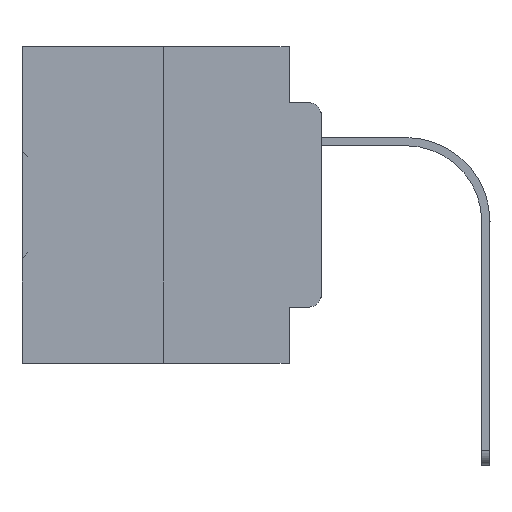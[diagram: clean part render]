
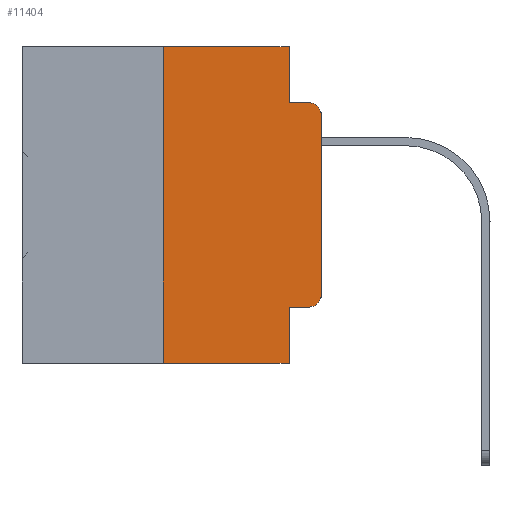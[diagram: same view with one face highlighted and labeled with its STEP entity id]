
A CAD part, left-side view. The second image highlights one B-rep face of the part: STEP entity #11404.
In plain terms, the highlighted planar face has unit normal (-1, 0, 0).
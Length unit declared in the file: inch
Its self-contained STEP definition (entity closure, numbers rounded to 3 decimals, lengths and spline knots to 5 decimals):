
#1369 = VECTOR ( 'NONE', #29465, 39.37008 ) ;
#1592 = EDGE_LOOP ( 'NONE', ( #9720, #23627, #23996, #33310, #8574, #29688, #16729, #21457, #33225, #32829 ) ) ;
#2369 = FACE_OUTER_BOUND ( 'NONE', #1592, .T. ) ;
#3070 = CARTESIAN_POINT ( 'NONE',  ( 0., 0.051, 0. ) ) ;
#3433 = CARTESIAN_POINT ( 'NONE',  ( 0., 0.051, 0. ) ) ;
#3533 = VECTOR ( 'NONE', #20103, 39.37008 ) ;
#3686 = CARTESIAN_POINT ( 'NONE',  ( 0., 0.02, -0.4115 ) ) ;
#3806 = EDGE_CURVE ( 'NONE', #13517, #10653, #35312, .T. ) ;
#4000 = VERTEX_POINT ( 'NONE', #9889 ) ;
#4002 = VECTOR ( 'NONE', #21553, 39.37008 ) ;
#4173 = CARTESIAN_POINT ( 'NONE',  ( 0., 0., -0.1085 ) ) ;
#4905 = VERTEX_POINT ( 'NONE', #32427 ) ;
#5281 = LINE ( 'NONE', #16525, #11997 ) ;
#6023 = AXIS2_PLACEMENT_3D ( 'NONE', #13680, #24733, #10956 ) ;
#6158 = VERTEX_POINT ( 'NONE', #9984 ) ;
#6289 = CARTESIAN_POINT ( 'NONE',  ( 0., 0.02, -0.1085 ) ) ;
#6512 = VECTOR ( 'NONE', #34035, 39.37008 ) ;
#6672 = EDGE_CURVE ( 'NONE', #13517, #21693, #14036, .T. ) ;
#6678 = LINE ( 'NONE', #22989, #6512 ) ;
#6750 = DIRECTION ( 'NONE',  ( 0., -1., 0. ) ) ;
#7418 = VECTOR ( 'NONE', #19670, 39.37008 ) ;
#8278 = DIRECTION ( 'NONE',  ( 0., -1., 0. ) ) ;
#8574 = ORIENTED_EDGE ( 'NONE', *, *, #13498, .F. ) ;
#9720 = ORIENTED_EDGE ( 'NONE', *, *, #31535, .T. ) ;
#9889 = CARTESIAN_POINT ( 'NONE',  ( 0., 0.25, 0. ) ) ;
#9984 = CARTESIAN_POINT ( 'NONE',  ( 0., 0.051, -0.0885 ) ) ;
#10167 = CARTESIAN_POINT ( 'NONE',  ( 0., 0.473, 0. ) ) ;
#10286 = AXIS2_PLACEMENT_3D ( 'NONE', #6289, #14257, #28202 ) ;
#10653 = VERTEX_POINT ( 'NONE', #25094 ) ;
#10956 = DIRECTION ( 'NONE',  ( 0., 0., -1. ) ) ;
#11021 = VECTOR ( 'NONE', #6750, 39.37008 ) ;
#11404 = ADVANCED_FACE ( 'NONE', ( #2369 ), #35518, .F. ) ;
#11754 = LINE ( 'NONE', #3070, #3533 ) ;
#11997 = VECTOR ( 'NONE', #16167, 39.37008 ) ;
#12366 = EDGE_CURVE ( 'NONE', #21693, #4905, #32625, .T. ) ;
#12946 = VERTEX_POINT ( 'NONE', #4173 ) ;
#13192 = CIRCLE ( 'NONE', #10286, 0.02 ) ;
#13308 = CARTESIAN_POINT ( 'NONE',  ( 0., 0.25, -0.5 ) ) ;
#13498 = EDGE_CURVE ( 'NONE', #4000, #30580, #18973, .T. ) ;
#13517 = VERTEX_POINT ( 'NONE', #32186 ) ;
#13675 = CARTESIAN_POINT ( 'NONE',  ( 0., 0.051, -0.4115 ) ) ;
#13680 = CARTESIAN_POINT ( 'NONE',  ( 0., 0.02, -0.3915 ) ) ;
#14036 = LINE ( 'NONE', #13675, #7418 ) ;
#14257 = DIRECTION ( 'NONE',  ( -1., 0., 0. ) ) ;
#14641 = VERTEX_POINT ( 'NONE', #30665 ) ;
#15230 = VECTOR ( 'NONE', #8278, 39.37008 ) ;
#16167 = DIRECTION ( 'NONE',  ( 0., 0., 1. ) ) ;
#16291 = LINE ( 'NONE', #34294, #11021 ) ;
#16525 = CARTESIAN_POINT ( 'NONE',  ( 0., 0., 0. ) ) ;
#16698 = EDGE_CURVE ( 'NONE', #30580, #6158, #11754, .T. ) ;
#16729 = ORIENTED_EDGE ( 'NONE', *, *, #20619, .T. ) ;
#18274 = CARTESIAN_POINT ( 'NONE',  ( 0., 0.473, 0. ) ) ;
#18356 = EDGE_CURVE ( 'NONE', #6158, #14641, #27309, .T. ) ;
#18973 = LINE ( 'NONE', #18274, #1369 ) ;
#19670 = DIRECTION ( 'NONE',  ( 0., -1., 0. ) ) ;
#20103 = DIRECTION ( 'NONE',  ( 0., 0., -1. ) ) ;
#20619 = EDGE_CURVE ( 'NONE', #21469, #10653, #16291, .T. ) ;
#21457 = ORIENTED_EDGE ( 'NONE', *, *, #3806, .F. ) ;
#21469 = VERTEX_POINT ( 'NONE', #13308 ) ;
#21553 = DIRECTION ( 'NONE',  ( 0., 0., -1. ) ) ;
#21693 = VERTEX_POINT ( 'NONE', #3686 ) ;
#22989 = CARTESIAN_POINT ( 'NONE',  ( 0., 0.25, 0. ) ) ;
#23627 = ORIENTED_EDGE ( 'NONE', *, *, #33695, .T. ) ;
#23996 = ORIENTED_EDGE ( 'NONE', *, *, #18356, .F. ) ;
#24733 = DIRECTION ( 'NONE',  ( -1., 0., 0. ) ) ;
#25094 = CARTESIAN_POINT ( 'NONE',  ( 0., 0.051, -0.5 ) ) ;
#26348 = EDGE_CURVE ( 'NONE', #21469, #4000, #6678, .T. ) ;
#27309 = LINE ( 'NONE', #32741, #15230 ) ;
#28160 = AXIS2_PLACEMENT_3D ( 'NONE', #10167, #35338, #30062 ) ;
#28202 = DIRECTION ( 'NONE',  ( 0., 0., -1. ) ) ;
#29465 = DIRECTION ( 'NONE',  ( 0., -1., 0. ) ) ;
#29688 = ORIENTED_EDGE ( 'NONE', *, *, #26348, .F. ) ;
#30062 = DIRECTION ( 'NONE',  ( 0., 0., -1. ) ) ;
#30580 = VERTEX_POINT ( 'NONE', #3433 ) ;
#30665 = CARTESIAN_POINT ( 'NONE',  ( 0., 0.02, -0.0885 ) ) ;
#31535 = EDGE_CURVE ( 'NONE', #4905, #12946, #5281, .T. ) ;
#32186 = CARTESIAN_POINT ( 'NONE',  ( 0., 0.051, -0.4115 ) ) ;
#32427 = CARTESIAN_POINT ( 'NONE',  ( 0., 0., -0.3915 ) ) ;
#32625 = CIRCLE ( 'NONE', #6023, 0.02 ) ;
#32741 = CARTESIAN_POINT ( 'NONE',  ( 0., 0.051, -0.0885 ) ) ;
#32829 = ORIENTED_EDGE ( 'NONE', *, *, #12366, .T. ) ;
#33121 = CARTESIAN_POINT ( 'NONE',  ( 0., 0.051, 0. ) ) ;
#33225 = ORIENTED_EDGE ( 'NONE', *, *, #6672, .T. ) ;
#33310 = ORIENTED_EDGE ( 'NONE', *, *, #16698, .F. ) ;
#33695 = EDGE_CURVE ( 'NONE', #12946, #14641, #13192, .T. ) ;
#34035 = DIRECTION ( 'NONE',  ( 0., 0., 1. ) ) ;
#34294 = CARTESIAN_POINT ( 'NONE',  ( 0., 0.473, -0.5 ) ) ;
#35312 = LINE ( 'NONE', #33121, #4002 ) ;
#35338 = DIRECTION ( 'NONE',  ( 1., 0., 0. ) ) ;
#35518 = PLANE ( 'NONE',  #28160 ) ;
